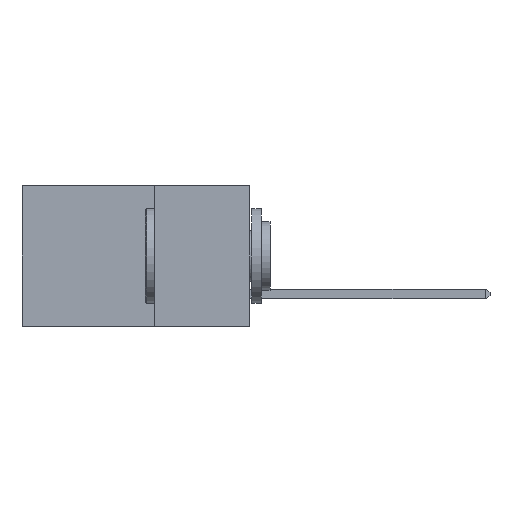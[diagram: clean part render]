
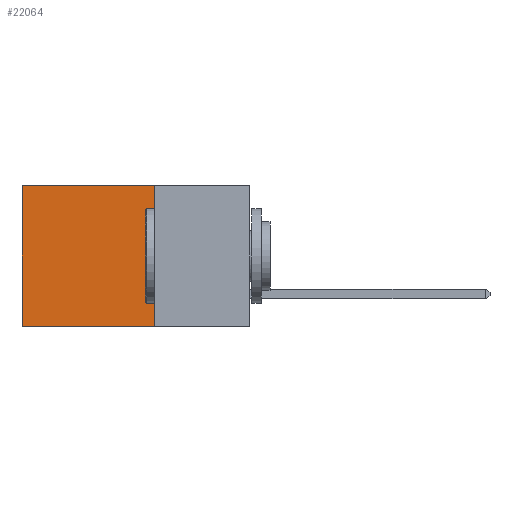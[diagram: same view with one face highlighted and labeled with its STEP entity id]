
A CAD part, left-side view. The second image highlights one B-rep face of the part: STEP entity #22064.
In plain terms, the highlighted planar face has unit normal (-1, 0, 0).
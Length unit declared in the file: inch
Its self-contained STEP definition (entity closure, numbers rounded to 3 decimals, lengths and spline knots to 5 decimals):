
#903 = CARTESIAN_POINT ( 'NONE',  ( 0.2875, 0.6, 0. ) ) ;
#3575 = VECTOR ( 'NONE', #11554, 39.37008 ) ;
#3908 = VERTEX_POINT ( 'NONE', #4034 ) ;
#4034 = CARTESIAN_POINT ( 'NONE',  ( 0.2875, 0.6, 0. ) ) ;
#4365 = ORIENTED_EDGE ( 'NONE', *, *, #10922, .F. ) ;
#4795 = VECTOR ( 'NONE', #15526, 39.37008 ) ;
#5779 = VECTOR ( 'NONE', #24611, 39.37008 ) ;
#6112 = CARTESIAN_POINT ( 'NONE',  ( 0.2875, 0.25, 0. ) ) ;
#6346 = CARTESIAN_POINT ( 'NONE',  ( 0.2875, 0.25, 0. ) ) ;
#6589 = EDGE_LOOP ( 'NONE', ( #14867, #4365, #26879, #28675 ) ) ;
#6598 = LINE ( 'NONE', #903, #5779 ) ;
#7175 = FACE_OUTER_BOUND ( 'NONE', #6589, .T. ) ;
#8897 = CARTESIAN_POINT ( 'NONE',  ( 0.2875, 0.25, 0. ) ) ;
#9052 = DIRECTION ( 'NONE',  ( 0., 0., -1. ) ) ;
#10922 = EDGE_CURVE ( 'NONE', #12171, #21348, #31143, .T. ) ;
#11554 = DIRECTION ( 'NONE',  ( 0., 1., 0. ) ) ;
#12171 = VERTEX_POINT ( 'NONE', #30956 ) ;
#13916 = CARTESIAN_POINT ( 'NONE',  ( 0.2875, 0.25, 0. ) ) ;
#14867 = ORIENTED_EDGE ( 'NONE', *, *, #18765, .T. ) ;
#15526 = DIRECTION ( 'NONE',  ( 0., 1., 0. ) ) ;
#17278 = LINE ( 'NONE', #13916, #32077 ) ;
#18138 = CARTESIAN_POINT ( 'NONE',  ( 0.2875, 0.25, -0.37 ) ) ;
#18377 = LINE ( 'NONE', #8897, #3575 ) ;
#18765 = EDGE_CURVE ( 'NONE', #3908, #21348, #6598, .T. ) ;
#19420 = PLANE ( 'NONE',  #32828 ) ;
#21348 = VERTEX_POINT ( 'NONE', #29687 ) ;
#22064 = ADVANCED_FACE ( 'NONE', ( #7175 ), #19420, .F. ) ;
#24611 = DIRECTION ( 'NONE',  ( 0., 0., -1. ) ) ;
#24777 = DIRECTION ( 'NONE',  ( 1., 0., 0. ) ) ;
#26568 = EDGE_CURVE ( 'NONE', #33130, #12171, #17278, .T. ) ;
#26879 = ORIENTED_EDGE ( 'NONE', *, *, #26568, .F. ) ;
#28675 = ORIENTED_EDGE ( 'NONE', *, *, #28733, .T. ) ;
#28733 = EDGE_CURVE ( 'NONE', #33130, #3908, #18377, .T. ) ;
#29687 = CARTESIAN_POINT ( 'NONE',  ( 0.2875, 0.6, -0.37 ) ) ;
#30956 = CARTESIAN_POINT ( 'NONE',  ( 0.2875, 0.25, -0.37 ) ) ;
#31143 = LINE ( 'NONE', #18138, #4795 ) ;
#32077 = VECTOR ( 'NONE', #32235, 39.37008 ) ;
#32235 = DIRECTION ( 'NONE',  ( 0., 0., -1. ) ) ;
#32828 = AXIS2_PLACEMENT_3D ( 'NONE', #6346, #24777, #9052 ) ;
#33130 = VERTEX_POINT ( 'NONE', #6112 ) ;
